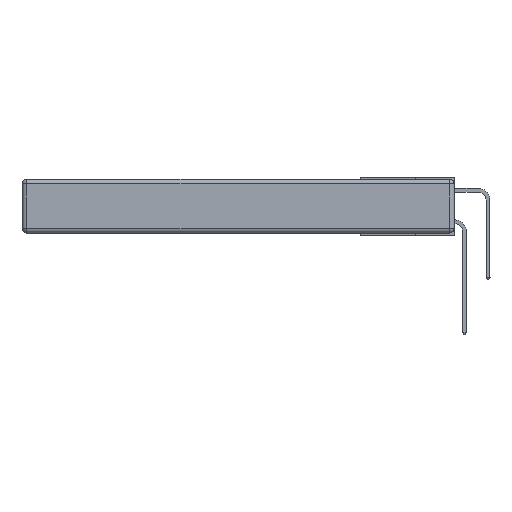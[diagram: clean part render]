
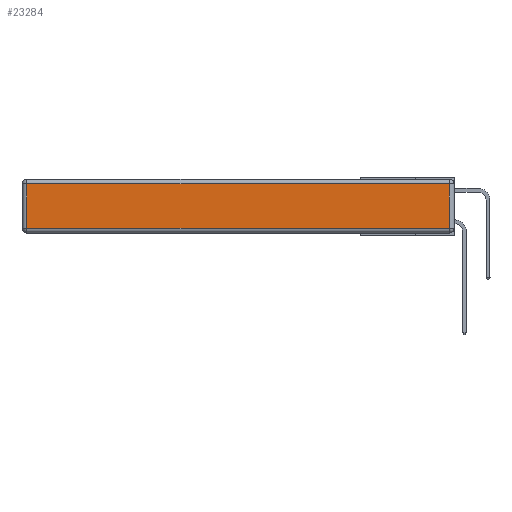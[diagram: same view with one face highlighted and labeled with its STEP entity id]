
A CAD part, left-side view. The second image highlights one B-rep face of the part: STEP entity #23284.
In plain terms, the highlighted planar face has unit normal (-1, 0, 0).
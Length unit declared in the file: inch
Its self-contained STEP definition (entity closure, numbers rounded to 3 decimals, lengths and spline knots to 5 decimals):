
#442 = CARTESIAN_POINT ( 'NONE',  ( 0., 2.72, -0.313 ) ) ;
#1405 = VECTOR ( 'NONE', #24052, 39.37008 ) ;
#1571 = CARTESIAN_POINT ( 'NONE',  ( 0., 2.72, -0.343 ) ) ;
#1855 = VECTOR ( 'NONE', #11232, 39.37008 ) ;
#1908 = PLANE ( 'NONE',  #11877 ) ;
#2078 = LINE ( 'NONE', #2082, #14606 ) ;
#2082 = CARTESIAN_POINT ( 'NONE',  ( 0., 0.03, -0.343 ) ) ;
#2887 = FACE_OUTER_BOUND ( 'NONE', #19875, .T. ) ;
#3089 = VERTEX_POINT ( 'NONE', #8433 ) ;
#3470 = ORIENTED_EDGE ( 'NONE', *, *, #19747, .T. ) ;
#5157 = EDGE_CURVE ( 'NONE', #7650, #3089, #7587, .T. ) ;
#7096 = DIRECTION ( 'NONE',  ( 0., 0., -1. ) ) ;
#7505 = EDGE_CURVE ( 'NONE', #17315, #7650, #2078, .T. ) ;
#7587 = LINE ( 'NONE', #19600, #1855 ) ;
#7650 = VERTEX_POINT ( 'NONE', #22029 ) ;
#8433 = CARTESIAN_POINT ( 'NONE',  ( 0., 2.72, -0.03 ) ) ;
#8599 = CARTESIAN_POINT ( 'NONE',  ( 0., 0., -0.343 ) ) ;
#8819 = VERTEX_POINT ( 'NONE', #442 ) ;
#11232 = DIRECTION ( 'NONE',  ( 0., 1., 0. ) ) ;
#11877 = AXIS2_PLACEMENT_3D ( 'NONE', #8599, #15117, #16837 ) ;
#12117 = CARTESIAN_POINT ( 'NONE',  ( 0., 0.03, -0.313 ) ) ;
#12551 = CARTESIAN_POINT ( 'NONE',  ( 0., 0., -0.313 ) ) ;
#12591 = ORIENTED_EDGE ( 'NONE', *, *, #7505, .T. ) ;
#12621 = ORIENTED_EDGE ( 'NONE', *, *, #18949, .T. ) ;
#13145 = DIRECTION ( 'NONE',  ( 0., 0., 1. ) ) ;
#14606 = VECTOR ( 'NONE', #13145, 39.37008 ) ;
#14943 = LINE ( 'NONE', #12551, #1405 ) ;
#15117 = DIRECTION ( 'NONE',  ( -1., 0., 0. ) ) ;
#16837 = DIRECTION ( 'NONE',  ( 0., 0., 1. ) ) ;
#17315 = VERTEX_POINT ( 'NONE', #12117 ) ;
#18949 = EDGE_CURVE ( 'NONE', #3089, #8819, #19700, .T. ) ;
#19600 = CARTESIAN_POINT ( 'NONE',  ( 0., 2.75, -0.03 ) ) ;
#19700 = LINE ( 'NONE', #1571, #21068 ) ;
#19747 = EDGE_CURVE ( 'NONE', #8819, #17315, #14943, .T. ) ;
#19875 = EDGE_LOOP ( 'NONE', ( #3470, #12591, #23498, #12621 ) ) ;
#21068 = VECTOR ( 'NONE', #7096, 39.37008 ) ;
#22029 = CARTESIAN_POINT ( 'NONE',  ( 0., 0.03, -0.03 ) ) ;
#23284 = ADVANCED_FACE ( 'NONE', ( #2887 ), #1908, .T. ) ;
#23498 = ORIENTED_EDGE ( 'NONE', *, *, #5157, .T. ) ;
#24052 = DIRECTION ( 'NONE',  ( 0., -1., 0. ) ) ;
